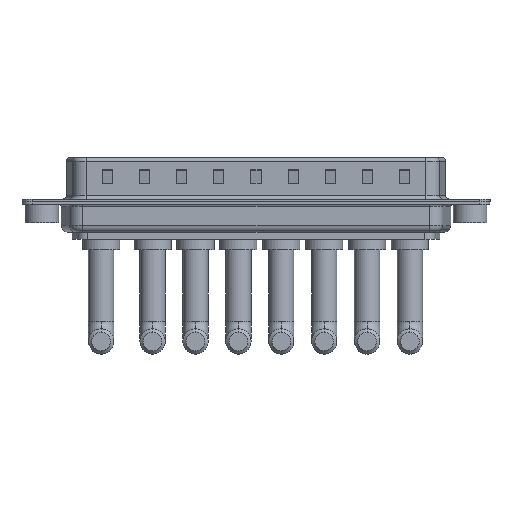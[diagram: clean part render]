
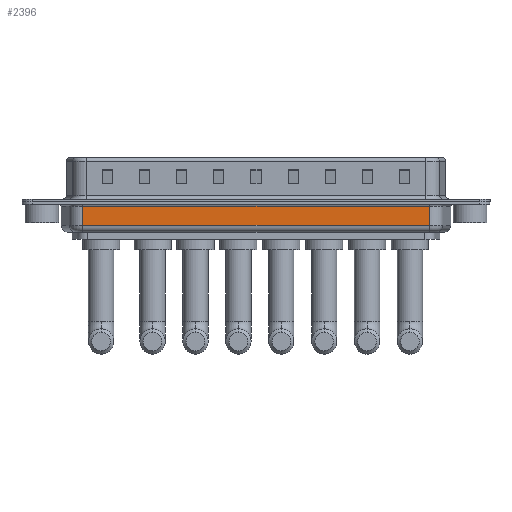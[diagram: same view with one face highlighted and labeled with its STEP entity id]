
A CAD part, front view. The second image highlights one B-rep face of the part: STEP entity #2396.
In plain terms, the highlighted planar face has unit normal (0, -1, 0).
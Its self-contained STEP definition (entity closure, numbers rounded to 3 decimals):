
#365 = VERTEX_POINT ( 'NONE', #14906 ) ;
#626 = CARTESIAN_POINT ( 'NONE',  ( 57.469, -5.35, -3.5 ) ) ;
#637 = VECTOR ( 'NONE', #15572, 1000. ) ;
#641 = VERTEX_POINT ( 'NONE', #10722 ) ;
#1165 = DIRECTION ( 'NONE',  ( 0., 0., 1. ) ) ;
#1170 = VERTEX_POINT ( 'NONE', #626 ) ;
#2396 = ADVANCED_FACE ( 'NONE', ( #9757 ), #7312, .F. ) ;
#2579 = VECTOR ( 'NONE', #6069, 1000. ) ;
#3081 = EDGE_CURVE ( 'NONE', #4175, #641, #9845, .T. ) ;
#3637 = CARTESIAN_POINT ( 'NONE',  ( 6.031, -5.35, -0.65 ) ) ;
#4175 = VERTEX_POINT ( 'NONE', #7672 ) ;
#4380 = LINE ( 'NONE', #4542, #637 ) ;
#4542 = CARTESIAN_POINT ( 'NONE',  ( 6.031, -5.35, -4.5 ) ) ;
#4830 = LINE ( 'NONE', #9976, #5112 ) ;
#5112 = VECTOR ( 'NONE', #1165, 1000. ) ;
#5773 = DIRECTION ( 'NONE',  ( -1., 0., 0. ) ) ;
#6069 = DIRECTION ( 'NONE',  ( 1., 0., 0. ) ) ;
#6497 = AXIS2_PLACEMENT_3D ( 'NONE', #8606, #14843, #7398 ) ;
#6893 = ORIENTED_EDGE ( 'NONE', *, *, #15139, .T. ) ;
#7290 = LINE ( 'NONE', #12266, #2579 ) ;
#7312 = PLANE ( 'NONE',  #6497 ) ;
#7398 = DIRECTION ( 'NONE',  ( -1., 0., 0. ) ) ;
#7672 = CARTESIAN_POINT ( 'NONE',  ( 57.469, -5.35, -0.65 ) ) ;
#8475 = EDGE_CURVE ( 'NONE', #365, #641, #4380, .T. ) ;
#8606 = CARTESIAN_POINT ( 'NONE',  ( 6.031, -5.35, -4.5 ) ) ;
#9066 = ORIENTED_EDGE ( 'NONE', *, *, #8475, .F. ) ;
#9130 = EDGE_LOOP ( 'NONE', ( #9066, #6893, #15350, #10869 ) ) ;
#9663 = VECTOR ( 'NONE', #5773, 1000. ) ;
#9757 = FACE_OUTER_BOUND ( 'NONE', #9130, .T. ) ;
#9845 = LINE ( 'NONE', #3637, #9663 ) ;
#9976 = CARTESIAN_POINT ( 'NONE',  ( 57.469, -5.35, -4.5 ) ) ;
#10722 = CARTESIAN_POINT ( 'NONE',  ( 6.031, -5.35, -0.65 ) ) ;
#10869 = ORIENTED_EDGE ( 'NONE', *, *, #3081, .T. ) ;
#11894 = EDGE_CURVE ( 'NONE', #1170, #4175, #4830, .T. ) ;
#12266 = CARTESIAN_POINT ( 'NONE',  ( 6.031, -5.35, -3.5 ) ) ;
#14843 = DIRECTION ( 'NONE',  ( 0., 1., 0. ) ) ;
#14906 = CARTESIAN_POINT ( 'NONE',  ( 6.031, -5.35, -3.5 ) ) ;
#15139 = EDGE_CURVE ( 'NONE', #365, #1170, #7290, .T. ) ;
#15350 = ORIENTED_EDGE ( 'NONE', *, *, #11894, .T. ) ;
#15572 = DIRECTION ( 'NONE',  ( 0., 0., 1. ) ) ;
